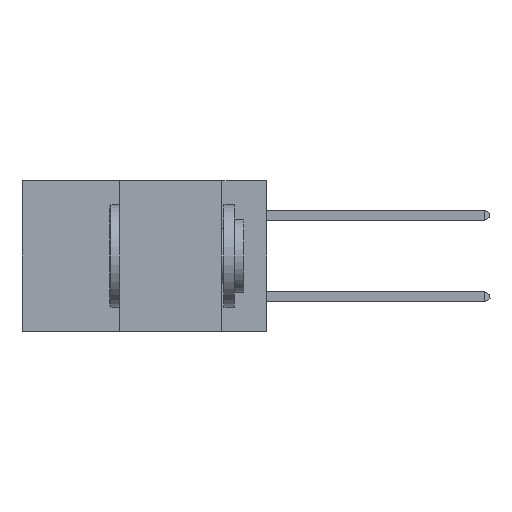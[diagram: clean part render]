
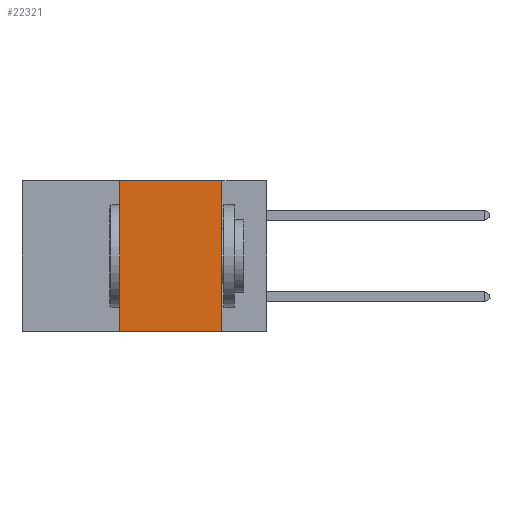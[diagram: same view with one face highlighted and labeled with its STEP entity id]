
A CAD part, left-side view. The second image highlights one B-rep face of the part: STEP entity #22321.
In plain terms, the highlighted planar face has unit normal (-1, 0, 0).
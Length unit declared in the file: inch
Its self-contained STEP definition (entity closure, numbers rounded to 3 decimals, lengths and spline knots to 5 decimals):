
#392 = CARTESIAN_POINT ( 'NONE',  ( 0., 0.11, 0. ) ) ;
#1341 = EDGE_CURVE ( 'NONE', #13887, #21782, #3424, .T. ) ;
#2337 = ORIENTED_EDGE ( 'NONE', *, *, #9451, .F. ) ;
#2343 = FACE_OUTER_BOUND ( 'NONE', #7320, .T. ) ;
#2511 = VECTOR ( 'NONE', #4886, 39.37008 ) ;
#3230 = DIRECTION ( 'NONE',  ( 1., 0., 0. ) ) ;
#3419 = LINE ( 'NONE', #5140, #12676 ) ;
#3424 = LINE ( 'NONE', #21900, #21442 ) ;
#4101 = AXIS2_PLACEMENT_3D ( 'NONE', #14290, #3230, #16072 ) ;
#4239 = CARTESIAN_POINT ( 'NONE',  ( 0., 0.6, 0. ) ) ;
#4267 = EDGE_CURVE ( 'NONE', #6548, #21782, #21693, .T. ) ;
#4886 = DIRECTION ( 'NONE',  ( 0., 0., -1. ) ) ;
#5140 = CARTESIAN_POINT ( 'NONE',  ( 0., 0.36, 0. ) ) ;
#5230 = ORIENTED_EDGE ( 'NONE', *, *, #21169, .F. ) ;
#6548 = VERTEX_POINT ( 'NONE', #392 ) ;
#6898 = PLANE ( 'NONE',  #4101 ) ;
#7241 = LINE ( 'NONE', #4239, #16363 ) ;
#7320 = EDGE_LOOP ( 'NONE', ( #12111, #2337, #5230, #20863 ) ) ;
#8889 = DIRECTION ( 'NONE',  ( 0., 0., 1. ) ) ;
#9451 = EDGE_CURVE ( 'NONE', #21392, #6548, #7241, .T. ) ;
#11704 = DIRECTION ( 'NONE',  ( 0., -1., 0. ) ) ;
#12111 = ORIENTED_EDGE ( 'NONE', *, *, #4267, .F. ) ;
#12378 = CARTESIAN_POINT ( 'NONE',  ( 0., 0.11, -0.37 ) ) ;
#12676 = VECTOR ( 'NONE', #8889, 39.37008 ) ;
#13887 = VERTEX_POINT ( 'NONE', #16546 ) ;
#14290 = CARTESIAN_POINT ( 'NONE',  ( 0., 0.6, 0. ) ) ;
#16072 = DIRECTION ( 'NONE',  ( 0., 0., -1. ) ) ;
#16363 = VECTOR ( 'NONE', #11704, 39.37008 ) ;
#16546 = CARTESIAN_POINT ( 'NONE',  ( 0., 0.36, -0.37 ) ) ;
#16632 = CARTESIAN_POINT ( 'NONE',  ( 0., 0.36, 0. ) ) ;
#19787 = DIRECTION ( 'NONE',  ( 0., -1., 0. ) ) ;
#20863 = ORIENTED_EDGE ( 'NONE', *, *, #1341, .T. ) ;
#21169 = EDGE_CURVE ( 'NONE', #13887, #21392, #3419, .T. ) ;
#21392 = VERTEX_POINT ( 'NONE', #16632 ) ;
#21442 = VECTOR ( 'NONE', #19787, 39.37008 ) ;
#21693 = LINE ( 'NONE', #22869, #2511 ) ;
#21782 = VERTEX_POINT ( 'NONE', #12378 ) ;
#21900 = CARTESIAN_POINT ( 'NONE',  ( 0., 0.6, -0.37 ) ) ;
#22321 = ADVANCED_FACE ( 'NONE', ( #2343 ), #6898, .F. ) ;
#22869 = CARTESIAN_POINT ( 'NONE',  ( 0., 0.11, 0. ) ) ;
